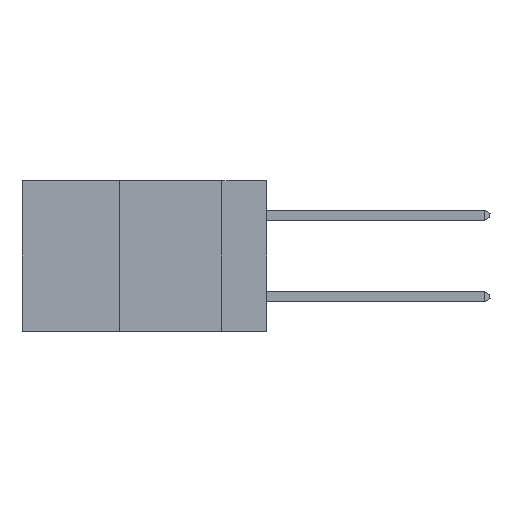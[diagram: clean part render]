
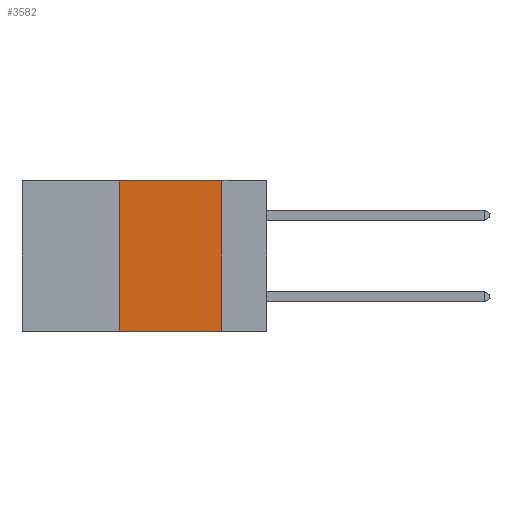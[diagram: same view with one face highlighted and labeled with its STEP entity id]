
A CAD part, left-side view. The second image highlights one B-rep face of the part: STEP entity #3582.
In plain terms, the highlighted planar face has unit normal (-1, 0, 0).
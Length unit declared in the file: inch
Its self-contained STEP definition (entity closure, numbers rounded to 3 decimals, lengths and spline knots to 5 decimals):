
#8 = LINE ( 'NONE', #1736, #17001 ) ;
#212 = DIRECTION ( 'NONE',  ( 0., 0., -1. ) ) ;
#1736 = CARTESIAN_POINT ( 'NONE',  ( 0., 0.6, -0.37 ) ) ;
#2259 = DIRECTION ( 'NONE',  ( 1., 0., 0. ) ) ;
#2438 = CARTESIAN_POINT ( 'NONE',  ( 0., 0.11, -0.37 ) ) ;
#3582 = ADVANCED_FACE ( 'NONE', ( #13184 ), #5679, .F. ) ;
#4919 = CARTESIAN_POINT ( 'NONE',  ( 0., 0.36, -0.37 ) ) ;
#5475 = ORIENTED_EDGE ( 'NONE', *, *, #9770, .F. ) ;
#5679 = PLANE ( 'NONE',  #13064 ) ;
#7247 = ORIENTED_EDGE ( 'NONE', *, *, #10234, .F. ) ;
#7947 = VERTEX_POINT ( 'NONE', #9867 ) ;
#9261 = ORIENTED_EDGE ( 'NONE', *, *, #20901, .F. ) ;
#9561 = LINE ( 'NONE', #18367, #20212 ) ;
#9763 = EDGE_LOOP ( 'NONE', ( #5475, #9261, #7247, #22003 ) ) ;
#9770 = EDGE_CURVE ( 'NONE', #19246, #17446, #9561, .T. ) ;
#9867 = CARTESIAN_POINT ( 'NONE',  ( 0., 0.36, 0. ) ) ;
#10234 = EDGE_CURVE ( 'NONE', #17477, #7947, #22095, .T. ) ;
#10250 = DIRECTION ( 'NONE',  ( 0., -1., 0. ) ) ;
#10613 = LINE ( 'NONE', #17839, #15553 ) ;
#12701 = CARTESIAN_POINT ( 'NONE',  ( 0., 0.6, 0. ) ) ;
#13064 = AXIS2_PLACEMENT_3D ( 'NONE', #12701, #2259, #212 ) ;
#13184 = FACE_OUTER_BOUND ( 'NONE', #9763, .T. ) ;
#14184 = EDGE_CURVE ( 'NONE', #17477, #17446, #8, .T. ) ;
#15074 = DIRECTION ( 'NONE',  ( 0., 0., -1. ) ) ;
#15369 = DIRECTION ( 'NONE',  ( 0., 0., 1. ) ) ;
#15553 = VECTOR ( 'NONE', #19577, 39.37008 ) ;
#17001 = VECTOR ( 'NONE', #10250, 39.37008 ) ;
#17139 = CARTESIAN_POINT ( 'NONE',  ( 0., 0.36, 0. ) ) ;
#17339 = CARTESIAN_POINT ( 'NONE',  ( 0., 0.11, 0. ) ) ;
#17446 = VERTEX_POINT ( 'NONE', #2438 ) ;
#17460 = VECTOR ( 'NONE', #15369, 39.37008 ) ;
#17477 = VERTEX_POINT ( 'NONE', #4919 ) ;
#17839 = CARTESIAN_POINT ( 'NONE',  ( 0., 0.6, 0. ) ) ;
#18367 = CARTESIAN_POINT ( 'NONE',  ( 0., 0.11, 0. ) ) ;
#19246 = VERTEX_POINT ( 'NONE', #17339 ) ;
#19577 = DIRECTION ( 'NONE',  ( 0., -1., 0. ) ) ;
#20212 = VECTOR ( 'NONE', #15074, 39.37008 ) ;
#20901 = EDGE_CURVE ( 'NONE', #7947, #19246, #10613, .T. ) ;
#22003 = ORIENTED_EDGE ( 'NONE', *, *, #14184, .T. ) ;
#22095 = LINE ( 'NONE', #17139, #17460 ) ;
